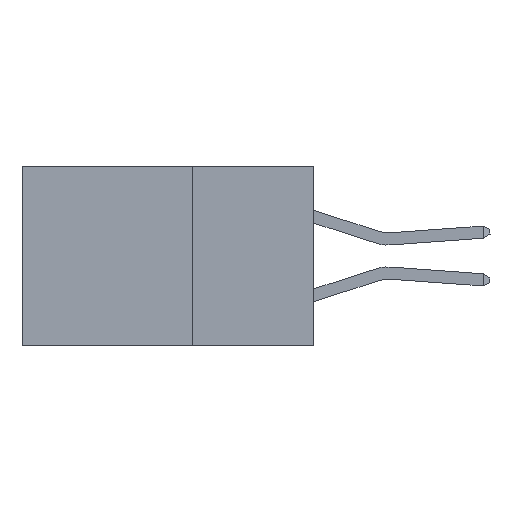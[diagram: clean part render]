
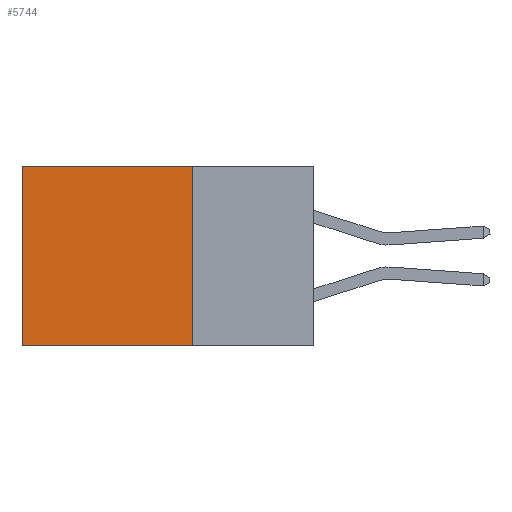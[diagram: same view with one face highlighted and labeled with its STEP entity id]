
A CAD part, left-side view. The second image highlights one B-rep face of the part: STEP entity #5744.
In plain terms, the highlighted planar face has unit normal (-1, 0, 0).
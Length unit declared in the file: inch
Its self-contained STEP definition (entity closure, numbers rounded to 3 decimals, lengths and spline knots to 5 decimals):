
#465 = LINE ( 'NONE', #8106, #15548 ) ;
#1034 = CARTESIAN_POINT ( 'NONE',  ( 0.2875, 0.25, -0.37 ) ) ;
#1298 = VECTOR ( 'NONE', #8335, 39.37008 ) ;
#1611 = DIRECTION ( 'NONE',  ( 0., 0., -1. ) ) ;
#2354 = CARTESIAN_POINT ( 'NONE',  ( 0.2875, 0.6, 0. ) ) ;
#2882 = DIRECTION ( 'NONE',  ( 1., 0., 0. ) ) ;
#4077 = FACE_OUTER_BOUND ( 'NONE', #11123, .T. ) ;
#4255 = LINE ( 'NONE', #6923, #1298 ) ;
#4320 = CARTESIAN_POINT ( 'NONE',  ( 0.2875, 0.25, 0. ) ) ;
#5050 = DIRECTION ( 'NONE',  ( 0., 0., -1. ) ) ;
#5489 = VERTEX_POINT ( 'NONE', #1034 ) ;
#5744 = ADVANCED_FACE ( 'NONE', ( #4077 ), #15870, .F. ) ;
#5905 = EDGE_CURVE ( 'NONE', #12938, #5489, #11482, .T. ) ;
#5963 = EDGE_CURVE ( 'NONE', #8695, #10858, #16540, .T. ) ;
#6436 = ORIENTED_EDGE ( 'NONE', *, *, #10500, .T. ) ;
#6923 = CARTESIAN_POINT ( 'NONE',  ( 0.2875, 0.25, -0.37 ) ) ;
#7021 = DIRECTION ( 'NONE',  ( 0., 1., 0. ) ) ;
#7200 = CARTESIAN_POINT ( 'NONE',  ( 0.2875, 0.6, -0.37 ) ) ;
#8106 = CARTESIAN_POINT ( 'NONE',  ( 0.2875, 0.25, 0. ) ) ;
#8335 = DIRECTION ( 'NONE',  ( 0., 1., 0. ) ) ;
#8695 = VERTEX_POINT ( 'NONE', #13584 ) ;
#10090 = ORIENTED_EDGE ( 'NONE', *, *, #5963, .T. ) ;
#10500 = EDGE_CURVE ( 'NONE', #12938, #8695, #465, .T. ) ;
#10858 = VERTEX_POINT ( 'NONE', #7200 ) ;
#11123 = EDGE_LOOP ( 'NONE', ( #10090, #14227, #15866, #6436 ) ) ;
#11153 = VECTOR ( 'NONE', #14080, 39.37008 ) ;
#11358 = CARTESIAN_POINT ( 'NONE',  ( 0.2875, 0.25, 0. ) ) ;
#11482 = LINE ( 'NONE', #16457, #11153 ) ;
#11864 = EDGE_CURVE ( 'NONE', #5489, #10858, #4255, .T. ) ;
#12938 = VERTEX_POINT ( 'NONE', #11358 ) ;
#13584 = CARTESIAN_POINT ( 'NONE',  ( 0.2875, 0.6, 0. ) ) ;
#14080 = DIRECTION ( 'NONE',  ( 0., 0., -1. ) ) ;
#14227 = ORIENTED_EDGE ( 'NONE', *, *, #11864, .F. ) ;
#14651 = VECTOR ( 'NONE', #5050, 39.37008 ) ;
#15548 = VECTOR ( 'NONE', #7021, 39.37008 ) ;
#15866 = ORIENTED_EDGE ( 'NONE', *, *, #5905, .F. ) ;
#15870 = PLANE ( 'NONE',  #16536 ) ;
#16457 = CARTESIAN_POINT ( 'NONE',  ( 0.2875, 0.25, 0. ) ) ;
#16536 = AXIS2_PLACEMENT_3D ( 'NONE', #4320, #2882, #1611 ) ;
#16540 = LINE ( 'NONE', #2354, #14651 ) ;
